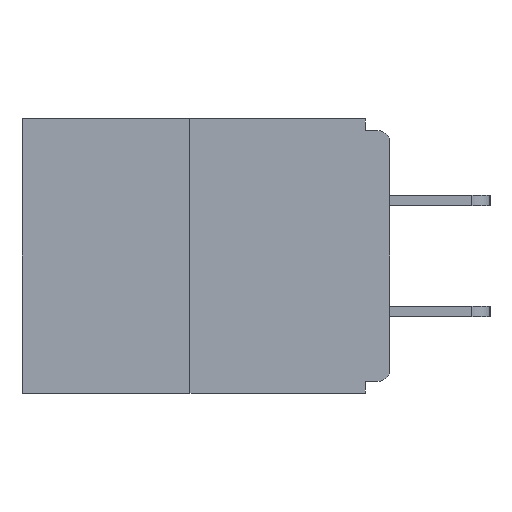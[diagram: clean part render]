
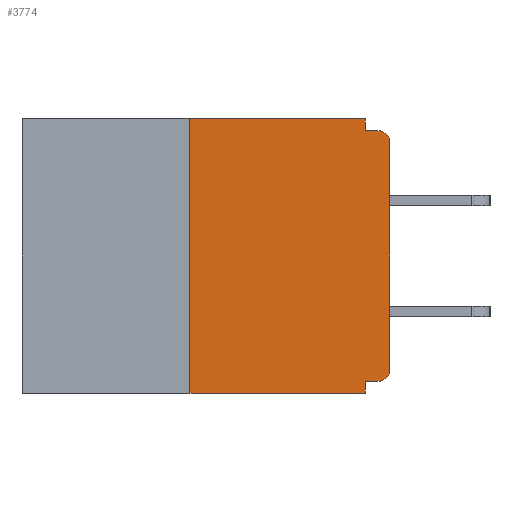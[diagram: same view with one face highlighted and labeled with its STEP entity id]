
A CAD part, left-side view. The second image highlights one B-rep face of the part: STEP entity #3774.
In plain terms, the highlighted planar face has unit normal (-1, 0, 0).
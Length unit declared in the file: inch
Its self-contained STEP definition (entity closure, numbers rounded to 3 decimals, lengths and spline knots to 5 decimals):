
#504 = CARTESIAN_POINT ( 'NONE',  ( 0., 0., -0.015 ) ) ;
#582 = LINE ( 'NONE', #6117, #6542 ) ;
#650 = CARTESIAN_POINT ( 'NONE',  ( 0., 0.46, 0. ) ) ;
#768 = LINE ( 'NONE', #12026, #3949 ) ;
#852 = ORIENTED_EDGE ( 'NONE', *, *, #11421, .T. ) ;
#1081 = ORIENTED_EDGE ( 'NONE', *, *, #2822, .F. ) ;
#1237 = CIRCLE ( 'NONE', #6737, 0.015 ) ;
#1395 = VECTOR ( 'NONE', #3209, 39.37008 ) ;
#1500 = LINE ( 'NONE', #7993, #8837 ) ;
#1521 = ORIENTED_EDGE ( 'NONE', *, *, #7202, .T. ) ;
#1535 = DIRECTION ( 'NONE',  ( 0., 0., -1. ) ) ;
#1568 = VERTEX_POINT ( 'NONE', #4877 ) ;
#1573 = DIRECTION ( 'NONE',  ( 0., 0., -1. ) ) ;
#1575 = AXIS2_PLACEMENT_3D ( 'NONE', #5285, #7131, #1535 ) ;
#1599 = ORIENTED_EDGE ( 'NONE', *, *, #8356, .T. ) ;
#1611 = EDGE_CURVE ( 'NONE', #6236, #11420, #3960, .T. ) ;
#1676 = ORIENTED_EDGE ( 'NONE', *, *, #1611, .F. ) ;
#2003 = CARTESIAN_POINT ( 'NONE',  ( 0., 0., -0.328 ) ) ;
#2141 = VECTOR ( 'NONE', #11754, 39.37008 ) ;
#2504 = DIRECTION ( 'NONE',  ( 1., 0., 0. ) ) ;
#2562 = DIRECTION ( 'NONE',  ( 0., 0., 1. ) ) ;
#2644 = LINE ( 'NONE', #12042, #5382 ) ;
#2822 = EDGE_CURVE ( 'NONE', #1568, #3816, #3648, .T. ) ;
#3023 = VERTEX_POINT ( 'NONE', #3081 ) ;
#3081 = CARTESIAN_POINT ( 'NONE',  ( 0., 0., -0.313 ) ) ;
#3209 = DIRECTION ( 'NONE',  ( 0., 0., 1. ) ) ;
#3284 = VERTEX_POINT ( 'NONE', #8282 ) ;
#3321 = VERTEX_POINT ( 'NONE', #9442 ) ;
#3370 = VECTOR ( 'NONE', #5631, 39.37008 ) ;
#3492 = DIRECTION ( 'NONE',  ( 0., 0., -1. ) ) ;
#3648 = LINE ( 'NONE', #504, #2141 ) ;
#3671 = ORIENTED_EDGE ( 'NONE', *, *, #6713, .F. ) ;
#3774 = ADVANCED_FACE ( 'NONE', ( #10908 ), #6295, .F. ) ;
#3816 = VERTEX_POINT ( 'NONE', #11211 ) ;
#3859 = LINE ( 'NONE', #6671, #3370 ) ;
#3949 = VECTOR ( 'NONE', #11085, 39.37008 ) ;
#3960 = LINE ( 'NONE', #2003, #9588 ) ;
#4280 = CARTESIAN_POINT ( 'NONE',  ( 0., 0.031, -0.343 ) ) ;
#4877 = CARTESIAN_POINT ( 'NONE',  ( 0., 0.031, -0.015 ) ) ;
#5285 = CARTESIAN_POINT ( 'NONE',  ( 0., 0.015, -0.03 ) ) ;
#5382 = VECTOR ( 'NONE', #10792, 39.37008 ) ;
#5631 = DIRECTION ( 'NONE',  ( 0., 0., -1. ) ) ;
#5670 = VERTEX_POINT ( 'NONE', #10218 ) ;
#5885 = LINE ( 'NONE', #9639, #1395 ) ;
#6117 = CARTESIAN_POINT ( 'NONE',  ( 0., 0.25, 0. ) ) ;
#6236 = VERTEX_POINT ( 'NONE', #10689 ) ;
#6295 = PLANE ( 'NONE',  #7055 ) ;
#6542 = VECTOR ( 'NONE', #2562, 39.37008 ) ;
#6671 = CARTESIAN_POINT ( 'NONE',  ( 0., 0.031, -0.343 ) ) ;
#6713 = EDGE_CURVE ( 'NONE', #3284, #5670, #2644, .T. ) ;
#6737 = AXIS2_PLACEMENT_3D ( 'NONE', #8942, #11772, #3492 ) ;
#7055 = AXIS2_PLACEMENT_3D ( 'NONE', #650, #2504, #1573 ) ;
#7131 = DIRECTION ( 'NONE',  ( -1., 0., 0. ) ) ;
#7149 = EDGE_CURVE ( 'NONE', #3321, #3284, #582, .T. ) ;
#7202 = EDGE_CURVE ( 'NONE', #6236, #3023, #1237, .T. ) ;
#7287 = CARTESIAN_POINT ( 'NONE',  ( 0., 0., -0.03 ) ) ;
#7455 = ORIENTED_EDGE ( 'NONE', *, *, #7623, .F. ) ;
#7623 = EDGE_CURVE ( 'NONE', #5670, #1568, #1500, .T. ) ;
#7624 = DIRECTION ( 'NONE',  ( 0., 1., 0. ) ) ;
#7993 = CARTESIAN_POINT ( 'NONE',  ( 0., 0.031, 0. ) ) ;
#8282 = CARTESIAN_POINT ( 'NONE',  ( 0., 0.25, 0. ) ) ;
#8356 = EDGE_CURVE ( 'NONE', #3023, #11359, #5885, .T. ) ;
#8404 = EDGE_CURVE ( 'NONE', #11359, #3816, #9213, .T. ) ;
#8837 = VECTOR ( 'NONE', #10829, 39.37008 ) ;
#8942 = CARTESIAN_POINT ( 'NONE',  ( 0., 0.015, -0.313 ) ) ;
#9154 = EDGE_CURVE ( 'NONE', #11420, #11820, #3859, .T. ) ;
#9180 = CARTESIAN_POINT ( 'NONE',  ( 0., 0.031, -0.328 ) ) ;
#9213 = CIRCLE ( 'NONE', #1575, 0.015 ) ;
#9366 = ORIENTED_EDGE ( 'NONE', *, *, #8404, .T. ) ;
#9442 = CARTESIAN_POINT ( 'NONE',  ( 0., 0.25, -0.343 ) ) ;
#9495 = ORIENTED_EDGE ( 'NONE', *, *, #7149, .F. ) ;
#9588 = VECTOR ( 'NONE', #7624, 39.37008 ) ;
#9639 = CARTESIAN_POINT ( 'NONE',  ( 0., 0., 0. ) ) ;
#10218 = CARTESIAN_POINT ( 'NONE',  ( 0., 0.031, 0. ) ) ;
#10618 = EDGE_LOOP ( 'NONE', ( #3671, #9495, #852, #11528, #1676, #1521, #1599, #9366, #1081, #7455 ) ) ;
#10689 = CARTESIAN_POINT ( 'NONE',  ( 0., 0.015, -0.328 ) ) ;
#10792 = DIRECTION ( 'NONE',  ( 0., -1., 0. ) ) ;
#10829 = DIRECTION ( 'NONE',  ( 0., 0., -1. ) ) ;
#10908 = FACE_OUTER_BOUND ( 'NONE', #10618, .T. ) ;
#11085 = DIRECTION ( 'NONE',  ( 0., -1., 0. ) ) ;
#11211 = CARTESIAN_POINT ( 'NONE',  ( 0., 0.015, -0.015 ) ) ;
#11359 = VERTEX_POINT ( 'NONE', #7287 ) ;
#11420 = VERTEX_POINT ( 'NONE', #9180 ) ;
#11421 = EDGE_CURVE ( 'NONE', #3321, #11820, #768, .T. ) ;
#11528 = ORIENTED_EDGE ( 'NONE', *, *, #9154, .F. ) ;
#11754 = DIRECTION ( 'NONE',  ( 0., -1., 0. ) ) ;
#11772 = DIRECTION ( 'NONE',  ( -1., 0., 0. ) ) ;
#11820 = VERTEX_POINT ( 'NONE', #4280 ) ;
#12026 = CARTESIAN_POINT ( 'NONE',  ( 0., 0.46, -0.343 ) ) ;
#12042 = CARTESIAN_POINT ( 'NONE',  ( 0., 0.46, 0. ) ) ;
